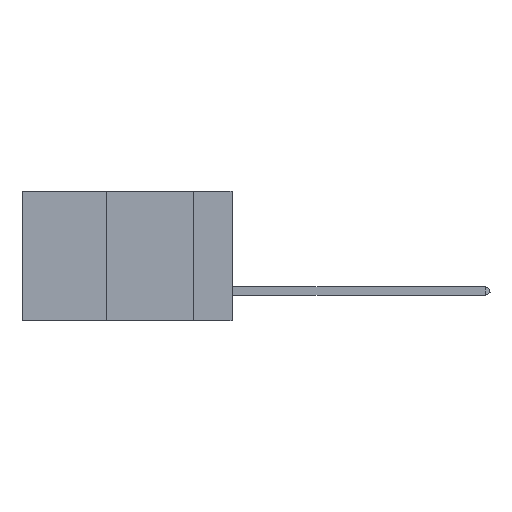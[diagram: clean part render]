
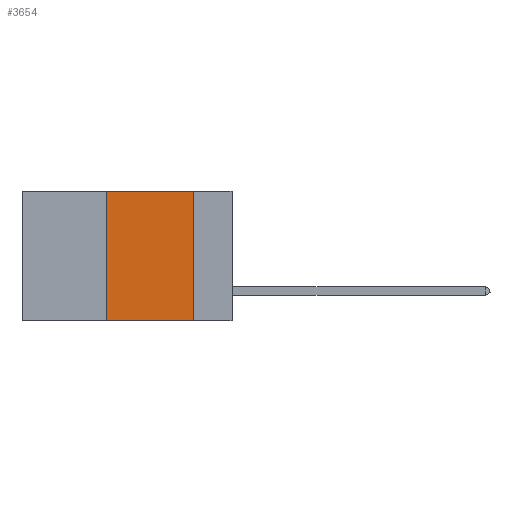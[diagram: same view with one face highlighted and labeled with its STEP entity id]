
A CAD part, left-side view. The second image highlights one B-rep face of the part: STEP entity #3654.
In plain terms, the highlighted planar face has unit normal (-1, 0, 0).
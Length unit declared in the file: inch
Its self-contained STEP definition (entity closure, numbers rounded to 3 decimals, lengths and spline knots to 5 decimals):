
#676 = VERTEX_POINT ( 'NONE', #14778 ) ;
#2335 = CARTESIAN_POINT ( 'NONE',  ( 0., 0.11, 0. ) ) ;
#3212 = ORIENTED_EDGE ( 'NONE', *, *, #15031, .F. ) ;
#3373 = LINE ( 'NONE', #13338, #4105 ) ;
#3435 = LINE ( 'NONE', #19036, #9813 ) ;
#3654 = ADVANCED_FACE ( 'NONE', ( #9795 ), #11825, .F. ) ;
#3725 = DIRECTION ( 'NONE',  ( 0., 0., -1. ) ) ;
#3976 = VERTEX_POINT ( 'NONE', #10747 ) ;
#4094 = AXIS2_PLACEMENT_3D ( 'NONE', #14935, #13573, #3725 ) ;
#4105 = VECTOR ( 'NONE', #19578, 39.37008 ) ;
#5093 = DIRECTION ( 'NONE',  ( 0., 0., -1. ) ) ;
#5656 = ORIENTED_EDGE ( 'NONE', *, *, #5871, .F. ) ;
#5726 = ORIENTED_EDGE ( 'NONE', *, *, #11157, .F. ) ;
#5870 = LINE ( 'NONE', #19777, #11512 ) ;
#5871 = EDGE_CURVE ( 'NONE', #9150, #676, #5870, .T. ) ;
#7515 = VECTOR ( 'NONE', #17226, 39.37008 ) ;
#8392 = VERTEX_POINT ( 'NONE', #18130 ) ;
#9150 = VERTEX_POINT ( 'NONE', #2335 ) ;
#9672 = ORIENTED_EDGE ( 'NONE', *, *, #21237, .T. ) ;
#9795 = FACE_OUTER_BOUND ( 'NONE', #14300, .T. ) ;
#9813 = VECTOR ( 'NONE', #14096, 39.37008 ) ;
#10747 = CARTESIAN_POINT ( 'NONE',  ( 0., 0.36, 0. ) ) ;
#11157 = EDGE_CURVE ( 'NONE', #8392, #3976, #3435, .T. ) ;
#11512 = VECTOR ( 'NONE', #5093, 39.37008 ) ;
#11825 = PLANE ( 'NONE',  #4094 ) ;
#13338 = CARTESIAN_POINT ( 'NONE',  ( 0., 0.6, -0.37 ) ) ;
#13573 = DIRECTION ( 'NONE',  ( 1., 0., 0. ) ) ;
#14096 = DIRECTION ( 'NONE',  ( 0., 0., 1. ) ) ;
#14300 = EDGE_LOOP ( 'NONE', ( #5656, #3212, #5726, #9672 ) ) ;
#14598 = CARTESIAN_POINT ( 'NONE',  ( 0., 0.6, 0. ) ) ;
#14778 = CARTESIAN_POINT ( 'NONE',  ( 0., 0.11, -0.37 ) ) ;
#14935 = CARTESIAN_POINT ( 'NONE',  ( 0., 0.6, 0. ) ) ;
#15031 = EDGE_CURVE ( 'NONE', #3976, #9150, #16512, .T. ) ;
#16512 = LINE ( 'NONE', #14598, #7515 ) ;
#17226 = DIRECTION ( 'NONE',  ( 0., -1., 0. ) ) ;
#18130 = CARTESIAN_POINT ( 'NONE',  ( 0., 0.36, -0.37 ) ) ;
#19036 = CARTESIAN_POINT ( 'NONE',  ( 0., 0.36, 0. ) ) ;
#19578 = DIRECTION ( 'NONE',  ( 0., -1., 0. ) ) ;
#19777 = CARTESIAN_POINT ( 'NONE',  ( 0., 0.11, 0. ) ) ;
#21237 = EDGE_CURVE ( 'NONE', #8392, #676, #3373, .T. ) ;
